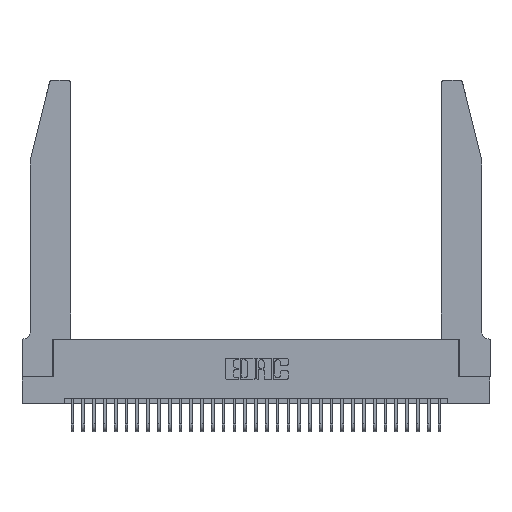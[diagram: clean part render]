
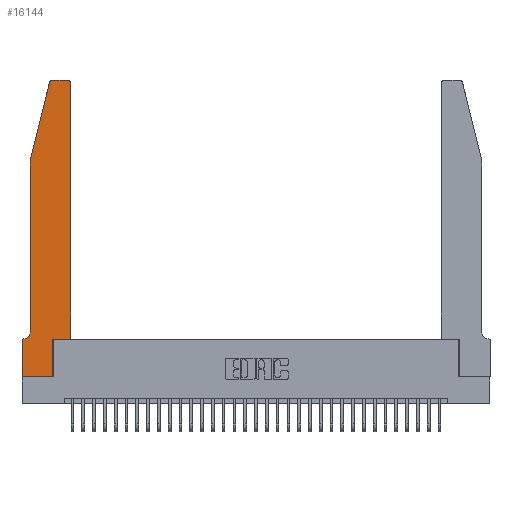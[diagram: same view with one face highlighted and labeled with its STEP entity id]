
A CAD part, top view. The second image highlights one B-rep face of the part: STEP entity #16144.
In plain terms, the highlighted planar face has unit normal (0, 0, 1).
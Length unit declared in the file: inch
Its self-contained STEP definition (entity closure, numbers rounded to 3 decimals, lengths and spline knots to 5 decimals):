
#2096 = ORIENTED_EDGE ( 'NONE', *, *, #18920, .T. ) ;
#2441 = VERTEX_POINT ( 'NONE', #24653 ) ;
#2504 = DIRECTION ( 'NONE',  ( 0., 0., 1. ) ) ;
#2721 = VERTEX_POINT ( 'NONE', #23007 ) ;
#2746 = CARTESIAN_POINT ( 'NONE',  ( 0.284, 2.75, 0.37 ) ) ;
#3277 = DIRECTION ( 'NONE',  ( 0., 0., 1. ) ) ;
#3734 = VERTEX_POINT ( 'NONE', #6298 ) ;
#4267 = CIRCLE ( 'NONE', #30573, 0.07 ) ;
#4389 = ORIENTED_EDGE ( 'NONE', *, *, #25463, .T. ) ;
#4450 = EDGE_CURVE ( 'NONE', #3734, #9682, #8895, .T. ) ;
#4645 = VECTOR ( 'NONE', #6183, 39.37008 ) ;
#6107 = VECTOR ( 'NONE', #14491, 39.37008 ) ;
#6183 = DIRECTION ( 'NONE',  ( 1., 0., 0. ) ) ;
#6202 = ORIENTED_EDGE ( 'NONE', *, *, #33880, .T. ) ;
#6298 = CARTESIAN_POINT ( 'NONE',  ( 0.4205, 2.75, 0.37 ) ) ;
#6368 = CARTESIAN_POINT ( 'NONE',  ( 0.2605, 2.75, 0.37 ) ) ;
#6499 = ORIENTED_EDGE ( 'NONE', *, *, #4450, .T. ) ;
#6534 = VECTOR ( 'NONE', #34802, 39.37008 ) ;
#7236 = VECTOR ( 'NONE', #25558, 39.37008 ) ;
#7936 = CARTESIAN_POINT ( 'NONE',  ( 0.25487, 2.72718, 0.37 ) ) ;
#8499 = CARTESIAN_POINT ( 'NONE',  ( 0.0755, 0.35, 0.37 ) ) ;
#8771 = EDGE_CURVE ( 'NONE', #28472, #18162, #20358, .T. ) ;
#8895 = LINE ( 'NONE', #6368, #22299 ) ;
#9103 = EDGE_LOOP ( 'NONE', ( #6499, #11072, #12751, #28025, #6202, #9839, #13264, #15084, #4389, #28717, #2096, #24632 ) ) ;
#9151 = CARTESIAN_POINT ( 'NONE',  ( 0.4505, 0.35, 0.37 ) ) ;
#9682 = VERTEX_POINT ( 'NONE', #2746 ) ;
#9839 = ORIENTED_EDGE ( 'NONE', *, *, #33259, .T. ) ;
#10392 = CARTESIAN_POINT ( 'NONE',  ( 0.4205, 2.72, 0.37 ) ) ;
#10586 = CARTESIAN_POINT ( 'NONE',  ( 0., 0., 0.37 ) ) ;
#11072 = ORIENTED_EDGE ( 'NONE', *, *, #31410, .T. ) ;
#11459 = VECTOR ( 'NONE', #20230, 39.37008 ) ;
#12751 = ORIENTED_EDGE ( 'NONE', *, *, #23306, .T. ) ;
#13069 = DIRECTION ( 'NONE',  ( 1., 0., 0. ) ) ;
#13264 = ORIENTED_EDGE ( 'NONE', *, *, #31977, .T. ) ;
#13447 = CARTESIAN_POINT ( 'NONE',  ( 0.0055, 0.42, 0.37 ) ) ;
#13849 = CIRCLE ( 'NONE', #20101, 0.03 ) ;
#14284 = LINE ( 'NONE', #20185, #7236 ) ;
#14313 = FACE_OUTER_BOUND ( 'NONE', #9103, .T. ) ;
#14491 = DIRECTION ( 'NONE',  ( 0., 1., 0. ) ) ;
#14535 = CARTESIAN_POINT ( 'NONE',  ( 0.2865, 0.35, 0.37 ) ) ;
#15084 = ORIENTED_EDGE ( 'NONE', *, *, #8771, .T. ) ;
#15206 = LINE ( 'NONE', #30119, #28665 ) ;
#15525 = DIRECTION ( 'NONE',  ( 0., 1., 0. ) ) ;
#15609 = VECTOR ( 'NONE', #16561, 39.37008 ) ;
#15675 = EDGE_CURVE ( 'NONE', #2441, #2721, #15206, .T. ) ;
#16144 = ADVANCED_FACE ( 'NONE', ( #14313 ), #34661, .T. ) ;
#16172 = DIRECTION ( 'NONE',  ( -1., 0., 0. ) ) ;
#16561 = DIRECTION ( 'NONE',  ( -1., 0., 0. ) ) ;
#16827 = VERTEX_POINT ( 'NONE', #7936 ) ;
#17485 = CARTESIAN_POINT ( 'NONE',  ( 0.4505, 0.35, 0.37 ) ) ;
#17508 = CARTESIAN_POINT ( 'NONE',  ( 0., 0., 0.37 ) ) ;
#18162 = VERTEX_POINT ( 'NONE', #24905 ) ;
#18395 = LINE ( 'NONE', #28922, #19243 ) ;
#18684 = VERTEX_POINT ( 'NONE', #29687 ) ;
#18699 = VERTEX_POINT ( 'NONE', #19048 ) ;
#18920 = EDGE_CURVE ( 'NONE', #29461, #20359, #21224, .T. ) ;
#19048 = CARTESIAN_POINT ( 'NONE',  ( 0.0055, 0.35, 0.37 ) ) ;
#19243 = VECTOR ( 'NONE', #15525, 39.37008 ) ;
#19403 = CARTESIAN_POINT ( 'NONE',  ( 0.284, 2.72, 0.37 ) ) ;
#19432 = CARTESIAN_POINT ( 'NONE',  ( 0.4505, 2.72, 0.37 ) ) ;
#19749 = DIRECTION ( 'NONE',  ( -1., 0., 0. ) ) ;
#20101 = AXIS2_PLACEMENT_3D ( 'NONE', #10392, #29158, #13069 ) ;
#20185 = CARTESIAN_POINT ( 'NONE',  ( 0.0755, 2., 0.37 ) ) ;
#20230 = DIRECTION ( 'NONE',  ( 1., 0., 0. ) ) ;
#20358 = LINE ( 'NONE', #17508, #11459 ) ;
#20359 = VERTEX_POINT ( 'NONE', #19432 ) ;
#20410 = VERTEX_POINT ( 'NONE', #14535 ) ;
#21224 = LINE ( 'NONE', #9151, #6107 ) ;
#21325 = DIRECTION ( 'NONE',  ( 1., 0., 0. ) ) ;
#21635 = LINE ( 'NONE', #32114, #6534 ) ;
#22071 = DIRECTION ( 'NONE',  ( 1., 0., 0. ) ) ;
#22233 = CARTESIAN_POINT ( 'NONE',  ( 0.4505, 0.35, 0.37 ) ) ;
#22299 = VECTOR ( 'NONE', #19749, 39.37008 ) ;
#23007 = CARTESIAN_POINT ( 'NONE',  ( 0.0755, 0.42, 0.37 ) ) ;
#23306 = EDGE_CURVE ( 'NONE', #16827, #2441, #14284, .T. ) ;
#23548 = EDGE_CURVE ( 'NONE', #20359, #3734, #13849, .T. ) ;
#23866 = EDGE_CURVE ( 'NONE', #20410, #29461, #33168, .T. ) ;
#24632 = ORIENTED_EDGE ( 'NONE', *, *, #23548, .T. ) ;
#24653 = CARTESIAN_POINT ( 'NONE',  ( 0.0755, 2., 0.37 ) ) ;
#24905 = CARTESIAN_POINT ( 'NONE',  ( 0.2865, 0., 0.37 ) ) ;
#25044 = AXIS2_PLACEMENT_3D ( 'NONE', #29286, #2504, #21325 ) ;
#25463 = EDGE_CURVE ( 'NONE', #18162, #20410, #18395, .T. ) ;
#25558 = DIRECTION ( 'NONE',  ( -0.239, -0.971, 0. ) ) ;
#26287 = AXIS2_PLACEMENT_3D ( 'NONE', #19403, #3277, #22071 ) ;
#28025 = ORIENTED_EDGE ( 'NONE', *, *, #15675, .T. ) ;
#28472 = VERTEX_POINT ( 'NONE', #10586 ) ;
#28665 = VECTOR ( 'NONE', #32810, 39.37008 ) ;
#28717 = ORIENTED_EDGE ( 'NONE', *, *, #23866, .T. ) ;
#28922 = CARTESIAN_POINT ( 'NONE',  ( 0.2865, 0.35, 0.37 ) ) ;
#29158 = DIRECTION ( 'NONE',  ( 0., 0., 1. ) ) ;
#29286 = CARTESIAN_POINT ( 'NONE',  ( 0., 0.35, 0.37 ) ) ;
#29461 = VERTEX_POINT ( 'NONE', #17485 ) ;
#29687 = CARTESIAN_POINT ( 'NONE',  ( 0., 0.35, 0.37 ) ) ;
#30119 = CARTESIAN_POINT ( 'NONE',  ( 0.0755, 2., 0.37 ) ) ;
#30573 = AXIS2_PLACEMENT_3D ( 'NONE', #13447, #32242, #16172 ) ;
#30734 = LINE ( 'NONE', #8499, #15609 ) ;
#31410 = EDGE_CURVE ( 'NONE', #9682, #16827, #32983, .T. ) ;
#31977 = EDGE_CURVE ( 'NONE', #18684, #28472, #21635, .T. ) ;
#32114 = CARTESIAN_POINT ( 'NONE',  ( 0., 0., 0.37 ) ) ;
#32242 = DIRECTION ( 'NONE',  ( 0., 0., -1. ) ) ;
#32810 = DIRECTION ( 'NONE',  ( 0., -1., 0. ) ) ;
#32983 = CIRCLE ( 'NONE', #26287, 0.03 ) ;
#33168 = LINE ( 'NONE', #22233, #4645 ) ;
#33259 = EDGE_CURVE ( 'NONE', #18699, #18684, #30734, .T. ) ;
#33880 = EDGE_CURVE ( 'NONE', #2721, #18699, #4267, .T. ) ;
#34661 = PLANE ( 'NONE',  #25044 ) ;
#34802 = DIRECTION ( 'NONE',  ( 0., -1., 0. ) ) ;
